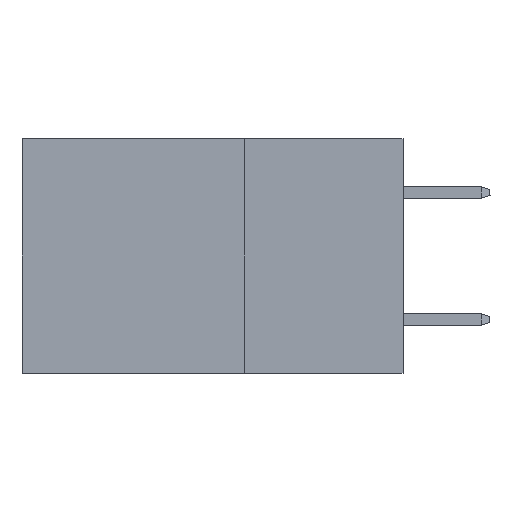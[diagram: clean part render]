
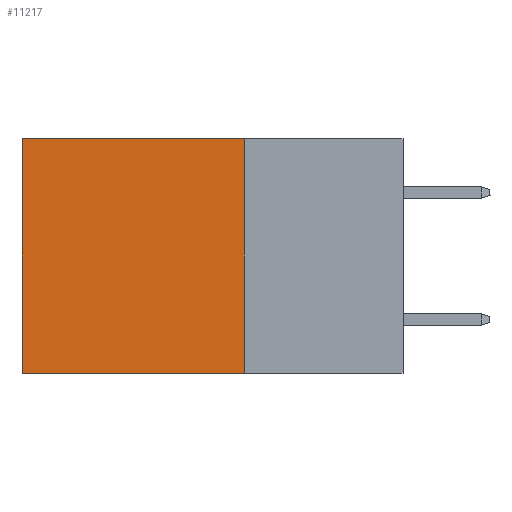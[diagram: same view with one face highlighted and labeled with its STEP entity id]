
A CAD part, left-side view. The second image highlights one B-rep face of the part: STEP entity #11217.
In plain terms, the highlighted planar face has unit normal (-1, 0, 0).
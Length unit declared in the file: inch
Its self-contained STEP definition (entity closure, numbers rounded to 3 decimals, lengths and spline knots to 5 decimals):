
#952 = LINE ( 'NONE', #6541, #12854 ) ;
#1121 = EDGE_CURVE ( 'NONE', #11370, #18428, #13151, .T. ) ;
#1776 = CARTESIAN_POINT ( 'NONE',  ( 0.2875, 0.6, -0.37 ) ) ;
#2494 = ORIENTED_EDGE ( 'NONE', *, *, #16226, .T. ) ;
#2922 = DIRECTION ( 'NONE',  ( 0., 0., -1. ) ) ;
#3003 = ORIENTED_EDGE ( 'NONE', *, *, #18642, .T. ) ;
#3778 = DIRECTION ( 'NONE',  ( 0., 1., 0. ) ) ;
#4032 = ORIENTED_EDGE ( 'NONE', *, *, #1121, .F. ) ;
#4054 = PLANE ( 'NONE',  #17123 ) ;
#5537 = CARTESIAN_POINT ( 'NONE',  ( 0.2875, 0.25, 0. ) ) ;
#5642 = CARTESIAN_POINT ( 'NONE',  ( 0.2875, 0.25, 0. ) ) ;
#6019 = EDGE_LOOP ( 'NONE', ( #3003, #21042, #4032, #2494 ) ) ;
#6541 = CARTESIAN_POINT ( 'NONE',  ( 0.2875, 0.6, 0. ) ) ;
#6677 = VECTOR ( 'NONE', #19244, 39.37008 ) ;
#6761 = CARTESIAN_POINT ( 'NONE',  ( 0.2875, 0.25, 0. ) ) ;
#8046 = CARTESIAN_POINT ( 'NONE',  ( 0.2875, 0.25, 0. ) ) ;
#9308 = DIRECTION ( 'NONE',  ( 0., 0., -1. ) ) ;
#10997 = DIRECTION ( 'NONE',  ( 1., 0., 0. ) ) ;
#11217 = ADVANCED_FACE ( 'NONE', ( #16269 ), #4054, .F. ) ;
#11306 = EDGE_CURVE ( 'NONE', #18428, #13614, #14483, .T. ) ;
#11370 = VERTEX_POINT ( 'NONE', #5537 ) ;
#12854 = VECTOR ( 'NONE', #13365, 39.37008 ) ;
#13043 = CARTESIAN_POINT ( 'NONE',  ( 0.2875, 0.6, 0. ) ) ;
#13151 = LINE ( 'NONE', #8046, #19928 ) ;
#13365 = DIRECTION ( 'NONE',  ( 0., 0., -1. ) ) ;
#13614 = VERTEX_POINT ( 'NONE', #1776 ) ;
#13709 = LINE ( 'NONE', #6761, #6677 ) ;
#14373 = CARTESIAN_POINT ( 'NONE',  ( 0.2875, 0.25, -0.37 ) ) ;
#14483 = LINE ( 'NONE', #14373, #20383 ) ;
#15707 = VERTEX_POINT ( 'NONE', #13043 ) ;
#16226 = EDGE_CURVE ( 'NONE', #11370, #15707, #13709, .T. ) ;
#16269 = FACE_OUTER_BOUND ( 'NONE', #6019, .T. ) ;
#17123 = AXIS2_PLACEMENT_3D ( 'NONE', #5642, #10997, #9308 ) ;
#17669 = CARTESIAN_POINT ( 'NONE',  ( 0.2875, 0.25, -0.37 ) ) ;
#18428 = VERTEX_POINT ( 'NONE', #17669 ) ;
#18642 = EDGE_CURVE ( 'NONE', #15707, #13614, #952, .T. ) ;
#19244 = DIRECTION ( 'NONE',  ( 0., 1., 0. ) ) ;
#19928 = VECTOR ( 'NONE', #2922, 39.37008 ) ;
#20383 = VECTOR ( 'NONE', #3778, 39.37008 ) ;
#21042 = ORIENTED_EDGE ( 'NONE', *, *, #11306, .F. ) ;
